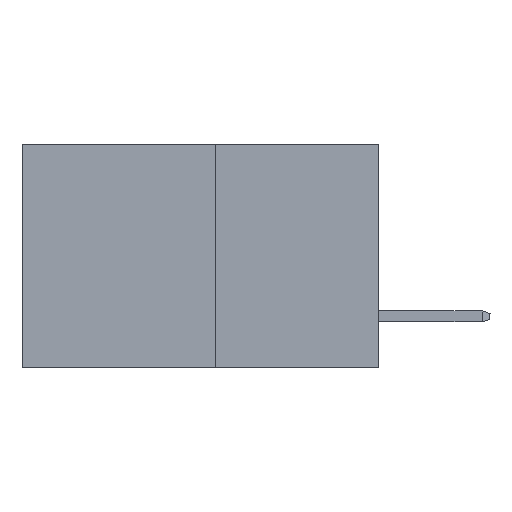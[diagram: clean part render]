
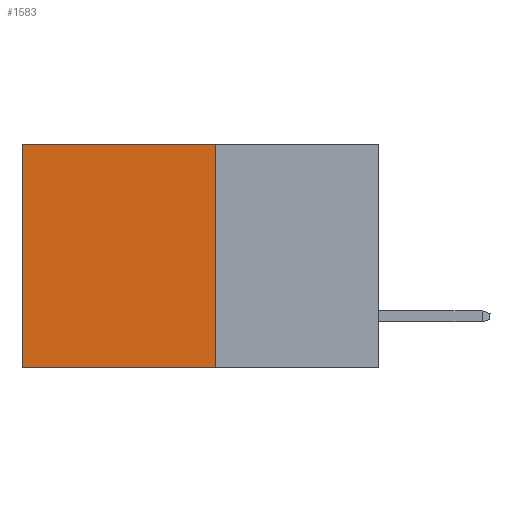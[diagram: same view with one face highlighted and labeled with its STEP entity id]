
A CAD part, left-side view. The second image highlights one B-rep face of the part: STEP entity #1583.
In plain terms, the highlighted planar face has unit normal (-1, 0, 0).
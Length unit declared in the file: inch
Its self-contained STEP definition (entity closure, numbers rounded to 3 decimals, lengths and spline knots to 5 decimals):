
#158 = ORIENTED_EDGE ( 'NONE', *, *, #12129, .F. ) ;
#172 = VECTOR ( 'NONE', #3915, 39.37008 ) ;
#414 = VERTEX_POINT ( 'NONE', #21584 ) ;
#1583 = ADVANCED_FACE ( 'NONE', ( #4985 ), #12811, .F. ) ;
#2605 = ORIENTED_EDGE ( 'NONE', *, *, #25300, .T. ) ;
#2699 = DIRECTION ( 'NONE',  ( 1., 0., 0. ) ) ;
#2975 = DIRECTION ( 'NONE',  ( 0., 0., -1. ) ) ;
#3113 = VERTEX_POINT ( 'NONE', #6132 ) ;
#3915 = DIRECTION ( 'NONE',  ( 0., 1., 0. ) ) ;
#4256 = DIRECTION ( 'NONE',  ( 0., 0., -1. ) ) ;
#4985 = FACE_OUTER_BOUND ( 'NONE', #7773, .T. ) ;
#5652 = VECTOR ( 'NONE', #24550, 39.37008 ) ;
#6093 = VERTEX_POINT ( 'NONE', #18567 ) ;
#6122 = LINE ( 'NONE', #9878, #5652 ) ;
#6132 = CARTESIAN_POINT ( 'NONE',  ( 0.277, 0.27, 0. ) ) ;
#6252 = VERTEX_POINT ( 'NONE', #25328 ) ;
#7773 = EDGE_LOOP ( 'NONE', ( #2605, #8018, #158, #10687 ) ) ;
#8018 = ORIENTED_EDGE ( 'NONE', *, *, #18687, .F. ) ;
#9740 = LINE ( 'NONE', #14754, #14723 ) ;
#9878 = CARTESIAN_POINT ( 'NONE',  ( 0.277, 0.27, 0. ) ) ;
#9922 = VECTOR ( 'NONE', #26982, 39.37008 ) ;
#10125 = CARTESIAN_POINT ( 'NONE',  ( 0.277, 0.27, -0.37 ) ) ;
#10687 = ORIENTED_EDGE ( 'NONE', *, *, #15585, .T. ) ;
#12129 = EDGE_CURVE ( 'NONE', #3113, #6252, #26660, .T. ) ;
#12811 = PLANE ( 'NONE',  #25467 ) ;
#14723 = VECTOR ( 'NONE', #4256, 39.37008 ) ;
#14754 = CARTESIAN_POINT ( 'NONE',  ( 0.277, 0.59, -0.37 ) ) ;
#15585 = EDGE_CURVE ( 'NONE', #3113, #414, #6122, .T. ) ;
#18567 = CARTESIAN_POINT ( 'NONE',  ( 0.277, 0.59, -0.37 ) ) ;
#18687 = EDGE_CURVE ( 'NONE', #6252, #6093, #22537, .T. ) ;
#21584 = CARTESIAN_POINT ( 'NONE',  ( 0.277, 0.59, 0. ) ) ;
#22537 = LINE ( 'NONE', #10125, #172 ) ;
#24369 = CARTESIAN_POINT ( 'NONE',  ( 0.277, 0.27, -0.37 ) ) ;
#24550 = DIRECTION ( 'NONE',  ( 0., 1., 0. ) ) ;
#24893 = CARTESIAN_POINT ( 'NONE',  ( 0.277, 0.27, -0.37 ) ) ;
#25300 = EDGE_CURVE ( 'NONE', #414, #6093, #9740, .T. ) ;
#25328 = CARTESIAN_POINT ( 'NONE',  ( 0.277, 0.27, -0.37 ) ) ;
#25467 = AXIS2_PLACEMENT_3D ( 'NONE', #24369, #2699, #2975 ) ;
#26660 = LINE ( 'NONE', #24893, #9922 ) ;
#26982 = DIRECTION ( 'NONE',  ( 0., 0., -1. ) ) ;
